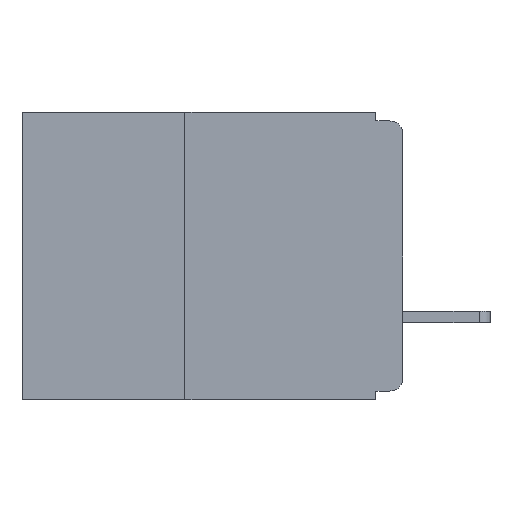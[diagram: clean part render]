
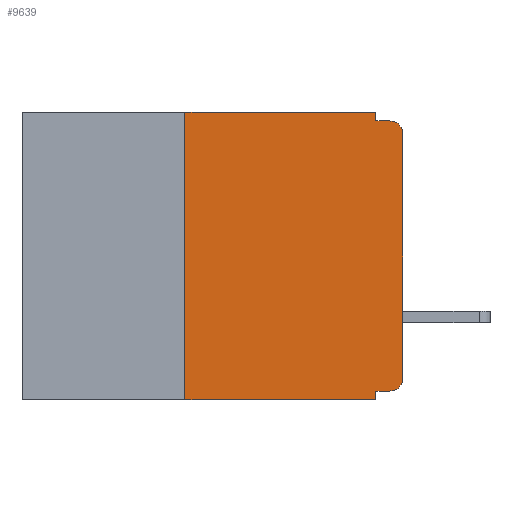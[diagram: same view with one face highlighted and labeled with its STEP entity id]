
A CAD part, left-side view. The second image highlights one B-rep face of the part: STEP entity #9639.
In plain terms, the highlighted planar face has unit normal (-1, 0, 0).
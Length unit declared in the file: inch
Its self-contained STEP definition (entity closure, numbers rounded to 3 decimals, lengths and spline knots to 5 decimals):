
#529 = CARTESIAN_POINT ( 'NONE',  ( 0., 0.25, -0.33 ) ) ;
#759 = CIRCLE ( 'NONE', #10676, 0.015 ) ;
#761 = CIRCLE ( 'NONE', #10748, 0.015 ) ;
#807 = CARTESIAN_POINT ( 'NONE',  ( 0., 0., -0.32 ) ) ;
#842 = VECTOR ( 'NONE', #3830, 39.37008 ) ;
#1083 = VECTOR ( 'NONE', #11878, 39.37008 ) ;
#1115 = LINE ( 'NONE', #807, #1083 ) ;
#1284 = VECTOR ( 'NONE', #1897, 39.37008 ) ;
#1362 = LINE ( 'NONE', #5843, #1284 ) ;
#1546 = VECTOR ( 'NONE', #4873, 39.37008 ) ;
#1897 = DIRECTION ( 'NONE',  ( 0., -1., 0. ) ) ;
#1909 = VECTOR ( 'NONE', #5991, 39.37008 ) ;
#1918 = VECTOR ( 'NONE', #6270, 39.37008 ) ;
#1951 = LINE ( 'NONE', #6074, #1918 ) ;
#2074 = CARTESIAN_POINT ( 'NONE',  ( 0., 0.031, -0.32 ) ) ;
#2131 = CARTESIAN_POINT ( 'NONE',  ( 0., 0.031, -0.01 ) ) ;
#2447 = CARTESIAN_POINT ( 'NONE',  ( 0., 0., -0.305 ) ) ;
#2748 = VERTEX_POINT ( 'NONE', #3682 ) ;
#3155 = VERTEX_POINT ( 'NONE', #2447 ) ;
#3270 = VECTOR ( 'NONE', #11694, 39.37008 ) ;
#3303 = LINE ( 'NONE', #10099, #3270 ) ;
#3341 = VERTEX_POINT ( 'NONE', #9813 ) ;
#3682 = CARTESIAN_POINT ( 'NONE',  ( 0., 0.015, -0.32 ) ) ;
#3744 = CARTESIAN_POINT ( 'NONE',  ( 0., 0.031, -0.33 ) ) ;
#3830 = DIRECTION ( 'NONE',  ( 0., 0., -1. ) ) ;
#4595 = ORIENTED_EDGE ( 'NONE', *, *, #6143, .F. ) ;
#4811 = ORIENTED_EDGE ( 'NONE', *, *, #5986, .F. ) ;
#4855 = ORIENTED_EDGE ( 'NONE', *, *, #7994, .F. ) ;
#4873 = DIRECTION ( 'NONE',  ( 0., -1., 0. ) ) ;
#4945 = ORIENTED_EDGE ( 'NONE', *, *, #6335, .T. ) ;
#5222 = CARTESIAN_POINT ( 'NONE',  ( 0., 0.437, -0.33 ) ) ;
#5303 = VERTEX_POINT ( 'NONE', #2074 ) ;
#5532 = DIRECTION ( 'NONE',  ( 0., 0., -1. ) ) ;
#5752 = AXIS2_PLACEMENT_3D ( 'NONE', #10028, #10741, #5532 ) ;
#5824 = DIRECTION ( 'NONE',  ( 0., 0., -1. ) ) ;
#5843 = CARTESIAN_POINT ( 'NONE',  ( 0., 0.437, 0. ) ) ;
#5854 = EDGE_CURVE ( 'NONE', #3155, #9826, #3303, .T. ) ;
#5986 = EDGE_CURVE ( 'NONE', #8734, #7648, #1951, .T. ) ;
#5991 = DIRECTION ( 'NONE',  ( 0., 0., 1. ) ) ;
#6029 = CARTESIAN_POINT ( 'NONE',  ( 0., 0.031, 0. ) ) ;
#6074 = CARTESIAN_POINT ( 'NONE',  ( 0., 0., -0.01 ) ) ;
#6143 = EDGE_CURVE ( 'NONE', #3341, #6402, #1362, .T. ) ;
#6165 = ORIENTED_EDGE ( 'NONE', *, *, #6385, .T. ) ;
#6210 = EDGE_CURVE ( 'NONE', #2748, #5303, #1115, .T. ) ;
#6270 = DIRECTION ( 'NONE',  ( 0., -1., 0. ) ) ;
#6284 = FACE_OUTER_BOUND ( 'NONE', #11045, .T. ) ;
#6324 = LINE ( 'NONE', #3744, #842 ) ;
#6331 = CARTESIAN_POINT ( 'NONE',  ( 0., 0.25, -0.33 ) ) ;
#6335 = EDGE_CURVE ( 'NONE', #9826, #7648, #761, .T. ) ;
#6385 = EDGE_CURVE ( 'NONE', #2748, #3155, #759, .T. ) ;
#6402 = VERTEX_POINT ( 'NONE', #10520 ) ;
#6884 = ORIENTED_EDGE ( 'NONE', *, *, #5854, .T. ) ;
#7271 = VECTOR ( 'NONE', #5824, 39.37008 ) ;
#7578 = LINE ( 'NONE', #6029, #7271 ) ;
#7648 = VERTEX_POINT ( 'NONE', #11425 ) ;
#7994 = EDGE_CURVE ( 'NONE', #6402, #8734, #7578, .T. ) ;
#8012 = EDGE_CURVE ( 'NONE', #8403, #3341, #11628, .T. ) ;
#8054 = EDGE_CURVE ( 'NONE', #8403, #9139, #9320, .T. ) ;
#8090 = EDGE_CURVE ( 'NONE', #5303, #9139, #6324, .T. ) ;
#8175 = ORIENTED_EDGE ( 'NONE', *, *, #6210, .F. ) ;
#8188 = ORIENTED_EDGE ( 'NONE', *, *, #8090, .F. ) ;
#8227 = CARTESIAN_POINT ( 'NONE',  ( 0., 0.031, -0.33 ) ) ;
#8287 = ORIENTED_EDGE ( 'NONE', *, *, #8054, .T. ) ;
#8403 = VERTEX_POINT ( 'NONE', #529 ) ;
#8632 = ORIENTED_EDGE ( 'NONE', *, *, #8012, .F. ) ;
#8734 = VERTEX_POINT ( 'NONE', #2131 ) ;
#9139 = VERTEX_POINT ( 'NONE', #8227 ) ;
#9230 = PLANE ( 'NONE',  #5752 ) ;
#9320 = LINE ( 'NONE', #5222, #1546 ) ;
#9639 = ADVANCED_FACE ( 'NONE', ( #6284 ), #9230, .F. ) ;
#9813 = CARTESIAN_POINT ( 'NONE',  ( 0., 0.25, 0. ) ) ;
#9826 = VERTEX_POINT ( 'NONE', #11491 ) ;
#10028 = CARTESIAN_POINT ( 'NONE',  ( 0., 0.437, 0. ) ) ;
#10099 = CARTESIAN_POINT ( 'NONE',  ( 0., 0., 0. ) ) ;
#10520 = CARTESIAN_POINT ( 'NONE',  ( 0., 0.031, 0. ) ) ;
#10676 = AXIS2_PLACEMENT_3D ( 'NONE', #10758, #10754, #10747 ) ;
#10741 = DIRECTION ( 'NONE',  ( 1., 0., 0. ) ) ;
#10747 = DIRECTION ( 'NONE',  ( 0., 0., -1. ) ) ;
#10748 = AXIS2_PLACEMENT_3D ( 'NONE', #11160, #11133, #11129 ) ;
#10754 = DIRECTION ( 'NONE',  ( -1., 0., 0. ) ) ;
#10758 = CARTESIAN_POINT ( 'NONE',  ( 0., 0.015, -0.305 ) ) ;
#11045 = EDGE_LOOP ( 'NONE', ( #6884, #4945, #4811, #4855, #4595, #8632, #8287, #8188, #8175, #6165 ) ) ;
#11129 = DIRECTION ( 'NONE',  ( 0., 0., -1. ) ) ;
#11133 = DIRECTION ( 'NONE',  ( -1., 0., 0. ) ) ;
#11160 = CARTESIAN_POINT ( 'NONE',  ( 0., 0.015, -0.025 ) ) ;
#11425 = CARTESIAN_POINT ( 'NONE',  ( 0., 0.015, -0.01 ) ) ;
#11491 = CARTESIAN_POINT ( 'NONE',  ( 0., 0., -0.025 ) ) ;
#11628 = LINE ( 'NONE', #6331, #1909 ) ;
#11694 = DIRECTION ( 'NONE',  ( 0., 0., 1. ) ) ;
#11878 = DIRECTION ( 'NONE',  ( 0., 1., 0. ) ) ;
